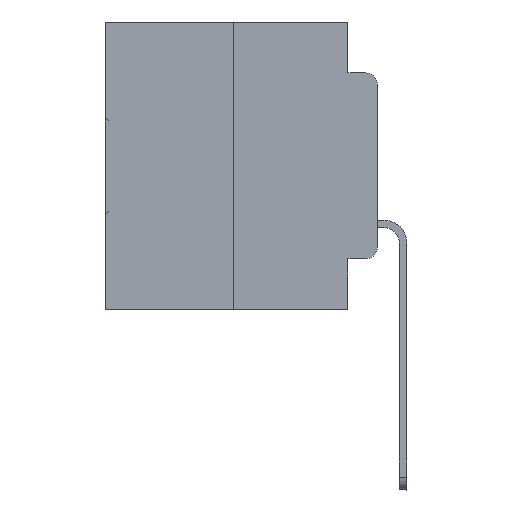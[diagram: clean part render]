
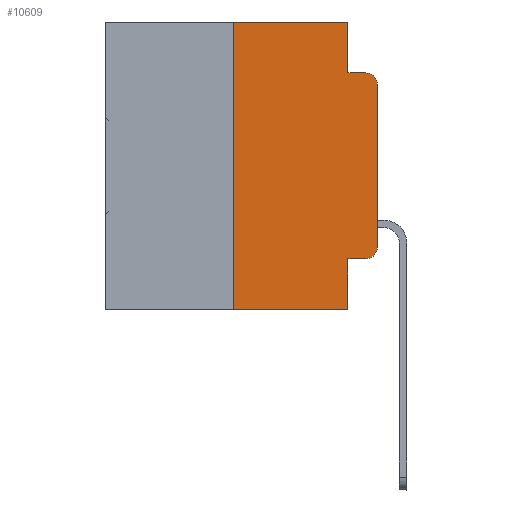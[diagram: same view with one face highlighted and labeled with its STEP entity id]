
A CAD part, left-side view. The second image highlights one B-rep face of the part: STEP entity #10609.
In plain terms, the highlighted planar face has unit normal (-1, 0, 0).
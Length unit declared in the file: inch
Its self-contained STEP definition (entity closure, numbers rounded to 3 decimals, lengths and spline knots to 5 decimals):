
#684 = LINE ( 'NONE', #14319, #17299 ) ;
#821 = EDGE_CURVE ( 'NONE', #17262, #3180, #22920, .T. ) ;
#823 = CARTESIAN_POINT ( 'NONE',  ( 0., 0., -0.1085 ) ) ;
#1015 = ORIENTED_EDGE ( 'NONE', *, *, #821, .F. ) ;
#1034 = CARTESIAN_POINT ( 'NONE',  ( 0., 0.051, -0.0885 ) ) ;
#1100 = CARTESIAN_POINT ( 'NONE',  ( 0., 0.051, 0. ) ) ;
#1384 = VECTOR ( 'NONE', #14644, 39.37008 ) ;
#1539 = CARTESIAN_POINT ( 'NONE',  ( 0., 0.051, 0. ) ) ;
#2507 = FACE_OUTER_BOUND ( 'NONE', #28061, .T. ) ;
#2797 = CARTESIAN_POINT ( 'NONE',  ( 0., 0.051, -0.5 ) ) ;
#3043 = DIRECTION ( 'NONE',  ( 0., 0., -1. ) ) ;
#3180 = VERTEX_POINT ( 'NONE', #10051 ) ;
#3455 = CIRCLE ( 'NONE', #5712, 0.02 ) ;
#4631 = LINE ( 'NONE', #1100, #28233 ) ;
#5407 = ORIENTED_EDGE ( 'NONE', *, *, #23912, .T. ) ;
#5700 = DIRECTION ( 'NONE',  ( -1., 0., 0. ) ) ;
#5712 = AXIS2_PLACEMENT_3D ( 'NONE', #29319, #5700, #3043 ) ;
#6947 = VERTEX_POINT ( 'NONE', #823 ) ;
#6952 = DIRECTION ( 'NONE',  ( 1., 0., 0. ) ) ;
#7759 = CARTESIAN_POINT ( 'NONE',  ( 0., 0.473, 0. ) ) ;
#8127 = LINE ( 'NONE', #15239, #14810 ) ;
#8327 = LINE ( 'NONE', #7759, #11656 ) ;
#8758 = EDGE_CURVE ( 'NONE', #28975, #18863, #32049, .T. ) ;
#9131 = ORIENTED_EDGE ( 'NONE', *, *, #33187, .F. ) ;
#10051 = CARTESIAN_POINT ( 'NONE',  ( 0., 0.02, -0.0885 ) ) ;
#10609 = ADVANCED_FACE ( 'NONE', ( #2507 ), #14642, .F. ) ;
#11656 = VECTOR ( 'NONE', #21104, 39.37008 ) ;
#11929 = VECTOR ( 'NONE', #33564, 39.37008 ) ;
#12088 = VERTEX_POINT ( 'NONE', #31908 ) ;
#12548 = VECTOR ( 'NONE', #24892, 39.37008 ) ;
#12678 = CARTESIAN_POINT ( 'NONE',  ( 0., 0., 0. ) ) ;
#12880 = ORIENTED_EDGE ( 'NONE', *, *, #15950, .F. ) ;
#13026 = CARTESIAN_POINT ( 'NONE',  ( 0., 0.02, -0.4115 ) ) ;
#13931 = CIRCLE ( 'NONE', #15847, 0.02 ) ;
#14120 = LINE ( 'NONE', #12678, #27757 ) ;
#14278 = CARTESIAN_POINT ( 'NONE',  ( 0., 0.051, 0. ) ) ;
#14319 = CARTESIAN_POINT ( 'NONE',  ( 0., 0.473, -0.5 ) ) ;
#14390 = CARTESIAN_POINT ( 'NONE',  ( 0., 0.051, -0.0885 ) ) ;
#14642 = PLANE ( 'NONE',  #19299 ) ;
#14644 = DIRECTION ( 'NONE',  ( 0., 0., -1. ) ) ;
#14810 = VECTOR ( 'NONE', #28980, 39.37008 ) ;
#15239 = CARTESIAN_POINT ( 'NONE',  ( 0., 0.25, 0. ) ) ;
#15847 = AXIS2_PLACEMENT_3D ( 'NONE', #24430, #29506, #18987 ) ;
#15950 = EDGE_CURVE ( 'NONE', #18765, #16176, #8327, .T. ) ;
#16176 = VERTEX_POINT ( 'NONE', #14278 ) ;
#16957 = ORIENTED_EDGE ( 'NONE', *, *, #25551, .T. ) ;
#17197 = DIRECTION ( 'NONE',  ( 0., 0., -1. ) ) ;
#17262 = VERTEX_POINT ( 'NONE', #14390 ) ;
#17299 = VECTOR ( 'NONE', #32847, 39.37008 ) ;
#18055 = EDGE_CURVE ( 'NONE', #28975, #25003, #19813, .T. ) ;
#18087 = CARTESIAN_POINT ( 'NONE',  ( 0., 0.25, 0. ) ) ;
#18765 = VERTEX_POINT ( 'NONE', #18087 ) ;
#18863 = VERTEX_POINT ( 'NONE', #2797 ) ;
#18987 = DIRECTION ( 'NONE',  ( 0., 0., -1. ) ) ;
#19299 = AXIS2_PLACEMENT_3D ( 'NONE', #22832, #6952, #17197 ) ;
#19813 = LINE ( 'NONE', #33449, #11929 ) ;
#20071 = CARTESIAN_POINT ( 'NONE',  ( 0., 0.051, -0.4115 ) ) ;
#21104 = DIRECTION ( 'NONE',  ( 0., -1., 0. ) ) ;
#22832 = CARTESIAN_POINT ( 'NONE',  ( 0., 0.473, 0. ) ) ;
#22920 = LINE ( 'NONE', #1034, #12548 ) ;
#23606 = ORIENTED_EDGE ( 'NONE', *, *, #18055, .T. ) ;
#23912 = EDGE_CURVE ( 'NONE', #33907, #6947, #14120, .T. ) ;
#24430 = CARTESIAN_POINT ( 'NONE',  ( 0., 0.02, -0.3915 ) ) ;
#24892 = DIRECTION ( 'NONE',  ( 0., -1., 0. ) ) ;
#25003 = VERTEX_POINT ( 'NONE', #13026 ) ;
#25521 = ORIENTED_EDGE ( 'NONE', *, *, #32230, .T. ) ;
#25551 = EDGE_CURVE ( 'NONE', #12088, #18863, #684, .T. ) ;
#26111 = DIRECTION ( 'NONE',  ( 0., 0., 1. ) ) ;
#26355 = ORIENTED_EDGE ( 'NONE', *, *, #27804, .T. ) ;
#26818 = CARTESIAN_POINT ( 'NONE',  ( 0., 0., -0.3915 ) ) ;
#27047 = ORIENTED_EDGE ( 'NONE', *, *, #8758, .F. ) ;
#27757 = VECTOR ( 'NONE', #26111, 39.37008 ) ;
#27804 = EDGE_CURVE ( 'NONE', #6947, #3180, #3455, .T. ) ;
#27815 = DIRECTION ( 'NONE',  ( 0., 0., -1. ) ) ;
#28061 = EDGE_LOOP ( 'NONE', ( #5407, #26355, #1015, #28884, #12880, #9131, #16957, #27047, #23606, #25521 ) ) ;
#28233 = VECTOR ( 'NONE', #27815, 39.37008 ) ;
#28743 = EDGE_CURVE ( 'NONE', #16176, #17262, #4631, .T. ) ;
#28884 = ORIENTED_EDGE ( 'NONE', *, *, #28743, .F. ) ;
#28975 = VERTEX_POINT ( 'NONE', #20071 ) ;
#28980 = DIRECTION ( 'NONE',  ( 0., 0., 1. ) ) ;
#29319 = CARTESIAN_POINT ( 'NONE',  ( 0., 0.02, -0.1085 ) ) ;
#29506 = DIRECTION ( 'NONE',  ( -1., 0., 0. ) ) ;
#31908 = CARTESIAN_POINT ( 'NONE',  ( 0., 0.25, -0.5 ) ) ;
#32049 = LINE ( 'NONE', #1539, #1384 ) ;
#32230 = EDGE_CURVE ( 'NONE', #25003, #33907, #13931, .T. ) ;
#32847 = DIRECTION ( 'NONE',  ( 0., -1., 0. ) ) ;
#33187 = EDGE_CURVE ( 'NONE', #12088, #18765, #8127, .T. ) ;
#33449 = CARTESIAN_POINT ( 'NONE',  ( 0., 0.051, -0.4115 ) ) ;
#33564 = DIRECTION ( 'NONE',  ( 0., -1., 0. ) ) ;
#33907 = VERTEX_POINT ( 'NONE', #26818 ) ;
